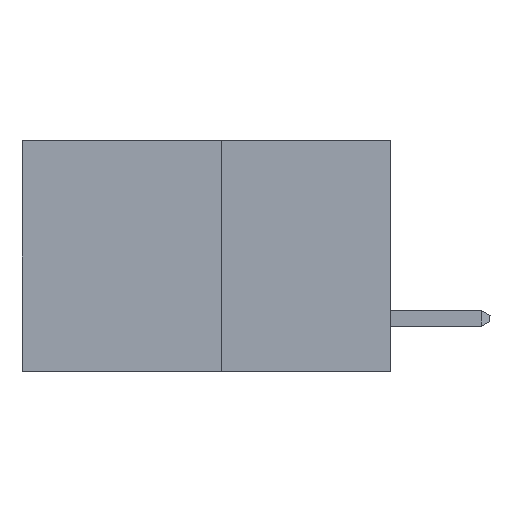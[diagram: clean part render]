
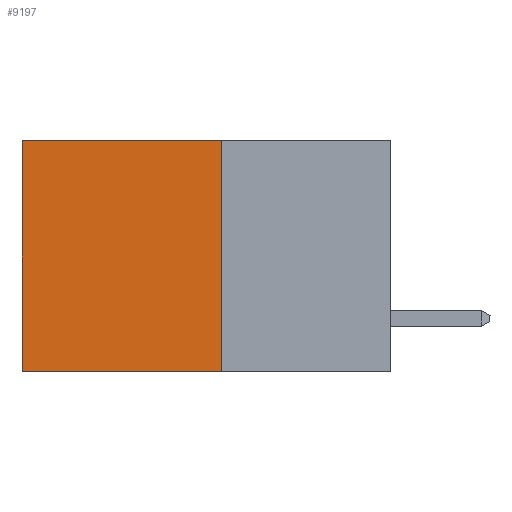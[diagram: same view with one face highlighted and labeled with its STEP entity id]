
A CAD part, left-side view. The second image highlights one B-rep face of the part: STEP entity #9197.
In plain terms, the highlighted planar face has unit normal (-1, 0, 0).
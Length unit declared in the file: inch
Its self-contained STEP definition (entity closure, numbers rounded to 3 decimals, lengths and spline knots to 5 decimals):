
#503 = CARTESIAN_POINT ( 'NONE',  ( 0.277, 0.27, 0. ) ) ;
#519 = EDGE_CURVE ( 'NONE', #7059, #3395, #10525, .T. ) ;
#688 = EDGE_LOOP ( 'NONE', ( #2898, #10682, #4055, #2612 ) ) ;
#885 = CARTESIAN_POINT ( 'NONE',  ( 0.277, 0.59, 0. ) ) ;
#1092 = EDGE_CURVE ( 'NONE', #7436, #7028, #11241, .T. ) ;
#1357 = CARTESIAN_POINT ( 'NONE',  ( 0.277, 0.27, -0.37 ) ) ;
#1400 = DIRECTION ( 'NONE',  ( 0., 0., -1. ) ) ;
#1603 = DIRECTION ( 'NONE',  ( 0., 1., 0. ) ) ;
#2612 = ORIENTED_EDGE ( 'NONE', *, *, #4355, .T. ) ;
#2898 = ORIENTED_EDGE ( 'NONE', *, *, #519, .T. ) ;
#3395 = VERTEX_POINT ( 'NONE', #9139 ) ;
#3760 = DIRECTION ( 'NONE',  ( 0., 0., -1. ) ) ;
#4055 = ORIENTED_EDGE ( 'NONE', *, *, #1092, .F. ) ;
#4147 = FACE_OUTER_BOUND ( 'NONE', #688, .T. ) ;
#4355 = EDGE_CURVE ( 'NONE', #7436, #7059, #10445, .T. ) ;
#5498 = VECTOR ( 'NONE', #1603, 39.37008 ) ;
#5969 = EDGE_CURVE ( 'NONE', #7028, #3395, #9657, .T. ) ;
#6220 = PLANE ( 'NONE',  #7410 ) ;
#6805 = DIRECTION ( 'NONE',  ( 0., 1., 0. ) ) ;
#6902 = DIRECTION ( 'NONE',  ( 0., 0., -1. ) ) ;
#7028 = VERTEX_POINT ( 'NONE', #11265 ) ;
#7059 = VERTEX_POINT ( 'NONE', #885 ) ;
#7145 = DIRECTION ( 'NONE',  ( 1., 0., 0. ) ) ;
#7410 = AXIS2_PLACEMENT_3D ( 'NONE', #1357, #7145, #1400 ) ;
#7436 = VERTEX_POINT ( 'NONE', #503 ) ;
#7670 = CARTESIAN_POINT ( 'NONE',  ( 0.277, 0.27, -0.37 ) ) ;
#8000 = CARTESIAN_POINT ( 'NONE',  ( 0.277, 0.27, -0.37 ) ) ;
#8022 = VECTOR ( 'NONE', #6902, 39.37008 ) ;
#8412 = CARTESIAN_POINT ( 'NONE',  ( 0.277, 0.27, 0. ) ) ;
#8732 = VECTOR ( 'NONE', #3760, 39.37008 ) ;
#9139 = CARTESIAN_POINT ( 'NONE',  ( 0.277, 0.59, -0.37 ) ) ;
#9197 = ADVANCED_FACE ( 'NONE', ( #4147 ), #6220, .F. ) ;
#9657 = LINE ( 'NONE', #7670, #11879 ) ;
#10445 = LINE ( 'NONE', #8412, #5498 ) ;
#10525 = LINE ( 'NONE', #10751, #8022 ) ;
#10682 = ORIENTED_EDGE ( 'NONE', *, *, #5969, .F. ) ;
#10751 = CARTESIAN_POINT ( 'NONE',  ( 0.277, 0.59, -0.37 ) ) ;
#11241 = LINE ( 'NONE', #8000, #8732 ) ;
#11265 = CARTESIAN_POINT ( 'NONE',  ( 0.277, 0.27, -0.37 ) ) ;
#11879 = VECTOR ( 'NONE', #6805, 39.37008 ) ;
